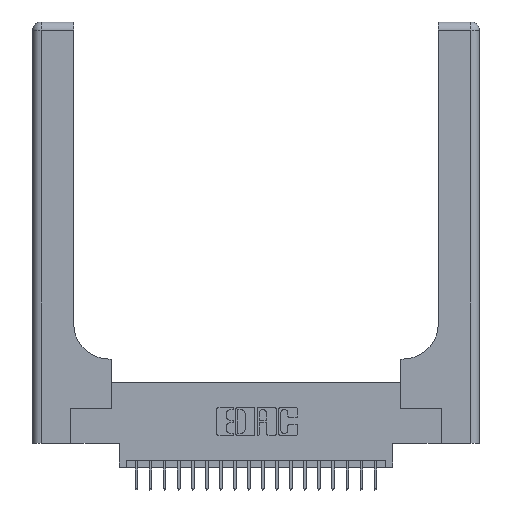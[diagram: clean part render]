
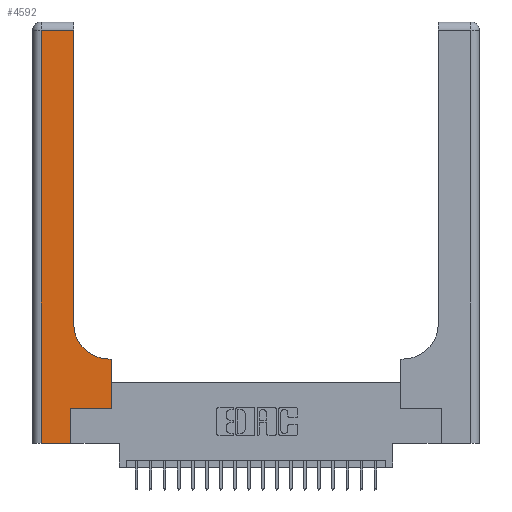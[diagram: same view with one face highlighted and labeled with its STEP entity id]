
A CAD part, top view. The second image highlights one B-rep face of the part: STEP entity #4592.
In plain terms, the highlighted planar face has unit normal (0, 0, 1).
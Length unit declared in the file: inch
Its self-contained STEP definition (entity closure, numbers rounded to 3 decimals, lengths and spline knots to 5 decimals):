
#26 = DIRECTION ( 'NONE',  ( -1., 0., 0. ) ) ;
#337 = LINE ( 'NONE', #3098, #22582 ) ;
#341 = DIRECTION ( 'NONE',  ( 0., 0., -1. ) ) ;
#718 = CARTESIAN_POINT ( 'NONE',  ( 0.5585, 0.25, 0.37 ) ) ;
#780 = LINE ( 'NONE', #11137, #14271 ) ;
#831 = CARTESIAN_POINT ( 'NONE',  ( 0.2915, 3., 0.37 ) ) ;
#1483 = DIRECTION ( 'NONE',  ( -1., 0., 0. ) ) ;
#1621 = VECTOR ( 'NONE', #22614, 39.37008 ) ;
#1703 = VERTEX_POINT ( 'NONE', #8587 ) ;
#1716 = CARTESIAN_POINT ( 'NONE',  ( 0.2915, 0.6, 0.37 ) ) ;
#1878 = ORIENTED_EDGE ( 'NONE', *, *, #11907, .T. ) ;
#2013 = ORIENTED_EDGE ( 'NONE', *, *, #8288, .T. ) ;
#2480 = AXIS2_PLACEMENT_3D ( 'NONE', #10152, #341, #3733 ) ;
#2622 = EDGE_CURVE ( 'NONE', #9548, #10555, #14443, .T. ) ;
#3064 = VERTEX_POINT ( 'NONE', #16567 ) ;
#3098 = CARTESIAN_POINT ( 'NONE',  ( 0., 2.94, 0.37 ) ) ;
#3263 = DIRECTION ( 'NONE',  ( 0., 0., -1. ) ) ;
#3661 = LINE ( 'NONE', #831, #21515 ) ;
#3733 = DIRECTION ( 'NONE',  ( -1., 0., 0. ) ) ;
#4280 = ORIENTED_EDGE ( 'NONE', *, *, #11468, .T. ) ;
#4426 = DIRECTION ( 'NONE',  ( 0., 1., 0. ) ) ;
#4592 = ADVANCED_FACE ( 'NONE', ( #11379 ), #10230, .F. ) ;
#4647 = CARTESIAN_POINT ( 'NONE',  ( 0.269, 0., 0.37 ) ) ;
#5072 = VECTOR ( 'NONE', #4426, 39.37008 ) ;
#5405 = EDGE_CURVE ( 'NONE', #3064, #9548, #17045, .T. ) ;
#6868 = DIRECTION ( 'NONE',  ( 1., 0., 0. ) ) ;
#7018 = ORIENTED_EDGE ( 'NONE', *, *, #9760, .T. ) ;
#7270 = DIRECTION ( 'NONE',  ( 1., 0., 0. ) ) ;
#8288 = EDGE_CURVE ( 'NONE', #19031, #22427, #12246, .T. ) ;
#8587 = CARTESIAN_POINT ( 'NONE',  ( 0.2915, 2.94, 0.37 ) ) ;
#9548 = VERTEX_POINT ( 'NONE', #11773 ) ;
#9647 = DIRECTION ( 'NONE',  ( 1., 0., 0. ) ) ;
#9753 = DIRECTION ( 'NONE',  ( 0., 1., 0. ) ) ;
#9760 = EDGE_CURVE ( 'NONE', #1703, #12232, #337, .T. ) ;
#10142 = LINE ( 'NONE', #12158, #1621 ) ;
#10152 = CARTESIAN_POINT ( 'NONE',  ( 0., 3., 0.37 ) ) ;
#10227 = ORIENTED_EDGE ( 'NONE', *, *, #2622, .T. ) ;
#10230 = PLANE ( 'NONE',  #2480 ) ;
#10333 = ORIENTED_EDGE ( 'NONE', *, *, #5405, .T. ) ;
#10555 = VERTEX_POINT ( 'NONE', #11534 ) ;
#10694 = CARTESIAN_POINT ( 'NONE',  ( 0., 0., 0.37 ) ) ;
#11137 = CARTESIAN_POINT ( 'NONE',  ( 0.269, 0., 0.37 ) ) ;
#11379 = FACE_OUTER_BOUND ( 'NONE', #16866, .T. ) ;
#11468 = EDGE_CURVE ( 'NONE', #21461, #14509, #22495, .T. ) ;
#11507 = CARTESIAN_POINT ( 'NONE',  ( 0.5415, 0.6, 0.37 ) ) ;
#11534 = CARTESIAN_POINT ( 'NONE',  ( 0.5585, 0.6, 0.37 ) ) ;
#11773 = CARTESIAN_POINT ( 'NONE',  ( 0.5585, 0.25, 0.37 ) ) ;
#11907 = EDGE_CURVE ( 'NONE', #12232, #21461, #10142, .T. ) ;
#12054 = CARTESIAN_POINT ( 'NONE',  ( 0.06, 0., 0.37 ) ) ;
#12158 = CARTESIAN_POINT ( 'NONE',  ( 0.06, 3., 0.37 ) ) ;
#12232 = VERTEX_POINT ( 'NONE', #20136 ) ;
#12246 = CIRCLE ( 'NONE', #20382, 0.25 ) ;
#12657 = VECTOR ( 'NONE', #7270, 39.37008 ) ;
#13188 = CARTESIAN_POINT ( 'NONE',  ( 0.269, 0.25, 0.37 ) ) ;
#13497 = CARTESIAN_POINT ( 'NONE',  ( 0.2915, 0.85, 0.37 ) ) ;
#13741 = CARTESIAN_POINT ( 'NONE',  ( 0.5415, 0.85, 0.37 ) ) ;
#14271 = VECTOR ( 'NONE', #21782, 39.37008 ) ;
#14443 = LINE ( 'NONE', #718, #5072 ) ;
#14509 = VERTEX_POINT ( 'NONE', #4647 ) ;
#15186 = VECTOR ( 'NONE', #26, 39.37008 ) ;
#15458 = LINE ( 'NONE', #1716, #15186 ) ;
#16480 = VECTOR ( 'NONE', #9647, 39.37008 ) ;
#16540 = ORIENTED_EDGE ( 'NONE', *, *, #22571, .T. ) ;
#16567 = CARTESIAN_POINT ( 'NONE',  ( 0.269, 0.25, 0.37 ) ) ;
#16866 = EDGE_LOOP ( 'NONE', ( #20513, #7018, #1878, #4280, #16540, #10333, #10227, #22286, #2013 ) ) ;
#17045 = LINE ( 'NONE', #13188, #16480 ) ;
#18787 = EDGE_CURVE ( 'NONE', #10555, #19031, #15458, .T. ) ;
#19031 = VERTEX_POINT ( 'NONE', #11507 ) ;
#19572 = EDGE_CURVE ( 'NONE', #22427, #1703, #3661, .T. ) ;
#20136 = CARTESIAN_POINT ( 'NONE',  ( 0.06, 2.94, 0.37 ) ) ;
#20382 = AXIS2_PLACEMENT_3D ( 'NONE', #13741, #3263, #6868 ) ;
#20513 = ORIENTED_EDGE ( 'NONE', *, *, #19572, .T. ) ;
#21461 = VERTEX_POINT ( 'NONE', #12054 ) ;
#21515 = VECTOR ( 'NONE', #9753, 39.37008 ) ;
#21782 = DIRECTION ( 'NONE',  ( 0., 1., 0. ) ) ;
#22286 = ORIENTED_EDGE ( 'NONE', *, *, #18787, .T. ) ;
#22427 = VERTEX_POINT ( 'NONE', #13497 ) ;
#22495 = LINE ( 'NONE', #10694, #12657 ) ;
#22571 = EDGE_CURVE ( 'NONE', #14509, #3064, #780, .T. ) ;
#22582 = VECTOR ( 'NONE', #1483, 39.37008 ) ;
#22614 = DIRECTION ( 'NONE',  ( 0., -1., 0. ) ) ;
